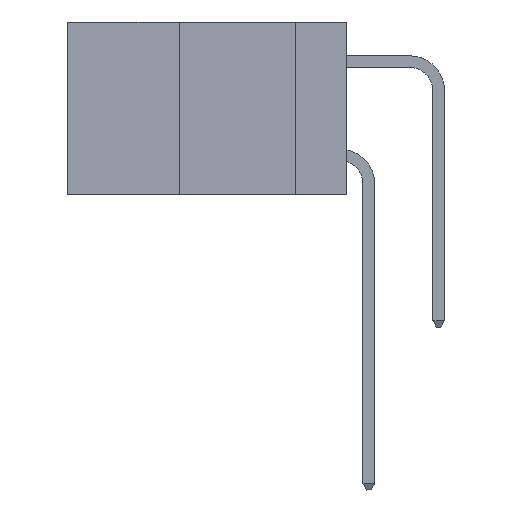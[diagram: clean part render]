
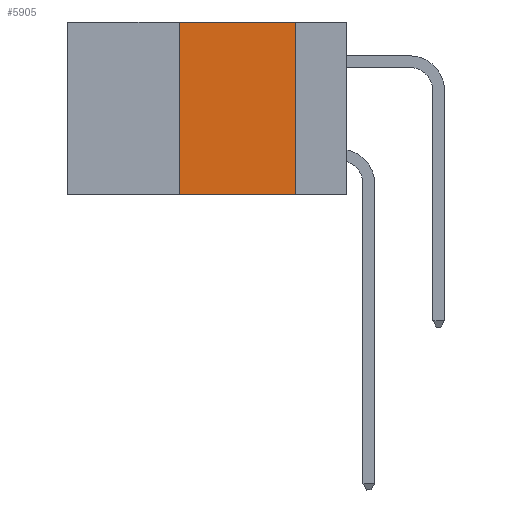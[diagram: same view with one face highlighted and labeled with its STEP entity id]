
A CAD part, left-side view. The second image highlights one B-rep face of the part: STEP entity #5905.
In plain terms, the highlighted planar face has unit normal (-1, 0, 0).
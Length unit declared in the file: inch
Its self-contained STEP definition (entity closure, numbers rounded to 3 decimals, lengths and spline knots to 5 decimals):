
#159 = AXIS2_PLACEMENT_3D ( 'NONE', #23378, #5907, #9713 ) ;
#299 = DIRECTION ( 'NONE',  ( 0., -1., 0. ) ) ;
#1067 = ORIENTED_EDGE ( 'NONE', *, *, #11192, .T. ) ;
#1508 = FACE_OUTER_BOUND ( 'NONE', #14608, .T. ) ;
#1559 = LINE ( 'NONE', #24517, #11368 ) ;
#3045 = CARTESIAN_POINT ( 'NONE',  ( 0., 0.36, 0. ) ) ;
#3159 = VERTEX_POINT ( 'NONE', #21448 ) ;
#5142 = EDGE_CURVE ( 'NONE', #16397, #3159, #1559, .T. ) ;
#5570 = CARTESIAN_POINT ( 'NONE',  ( 0., 0.11, 0. ) ) ;
#5905 = ADVANCED_FACE ( 'NONE', ( #1508 ), #17229, .F. ) ;
#5907 = DIRECTION ( 'NONE',  ( 1., 0., 0. ) ) ;
#6528 = DIRECTION ( 'NONE',  ( 0., 0., 1. ) ) ;
#7525 = CARTESIAN_POINT ( 'NONE',  ( 0., 0.6, -0.37 ) ) ;
#7607 = DIRECTION ( 'NONE',  ( 0., -1., 0. ) ) ;
#8356 = CARTESIAN_POINT ( 'NONE',  ( 0., 0.36, 0. ) ) ;
#8826 = ORIENTED_EDGE ( 'NONE', *, *, #11546, .F. ) ;
#9360 = LINE ( 'NONE', #7525, #21386 ) ;
#9713 = DIRECTION ( 'NONE',  ( 0., 0., -1. ) ) ;
#10169 = ORIENTED_EDGE ( 'NONE', *, *, #16072, .F. ) ;
#10459 = VERTEX_POINT ( 'NONE', #12606 ) ;
#11192 = EDGE_CURVE ( 'NONE', #14736, #10459, #9360, .T. ) ;
#11368 = VECTOR ( 'NONE', #299, 39.37008 ) ;
#11546 = EDGE_CURVE ( 'NONE', #3159, #10459, #20450, .T. ) ;
#12606 = CARTESIAN_POINT ( 'NONE',  ( 0., 0.11, -0.37 ) ) ;
#14608 = EDGE_LOOP ( 'NONE', ( #8826, #17489, #10169, #1067 ) ) ;
#14716 = VECTOR ( 'NONE', #17852, 39.37008 ) ;
#14736 = VERTEX_POINT ( 'NONE', #19059 ) ;
#14757 = VECTOR ( 'NONE', #6528, 39.37008 ) ;
#16072 = EDGE_CURVE ( 'NONE', #14736, #16397, #19211, .T. ) ;
#16397 = VERTEX_POINT ( 'NONE', #3045 ) ;
#17229 = PLANE ( 'NONE',  #159 ) ;
#17489 = ORIENTED_EDGE ( 'NONE', *, *, #5142, .F. ) ;
#17852 = DIRECTION ( 'NONE',  ( 0., 0., -1. ) ) ;
#19059 = CARTESIAN_POINT ( 'NONE',  ( 0., 0.36, -0.37 ) ) ;
#19211 = LINE ( 'NONE', #8356, #14757 ) ;
#20450 = LINE ( 'NONE', #5570, #14716 ) ;
#21386 = VECTOR ( 'NONE', #7607, 39.37008 ) ;
#21448 = CARTESIAN_POINT ( 'NONE',  ( 0., 0.11, 0. ) ) ;
#23378 = CARTESIAN_POINT ( 'NONE',  ( 0., 0.6, 0. ) ) ;
#24517 = CARTESIAN_POINT ( 'NONE',  ( 0., 0.6, 0. ) ) ;
